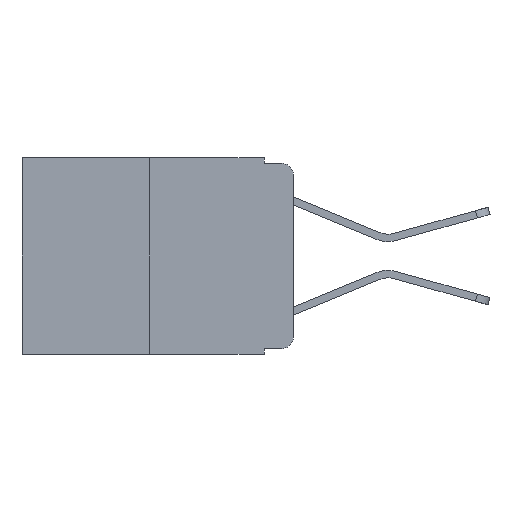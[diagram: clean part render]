
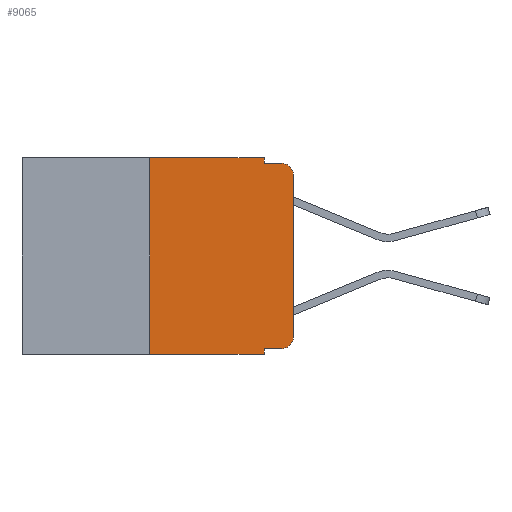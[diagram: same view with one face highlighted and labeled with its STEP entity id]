
A CAD part, left-side view. The second image highlights one B-rep face of the part: STEP entity #9065.
In plain terms, the highlighted planar face has unit normal (-1, 0, 0).
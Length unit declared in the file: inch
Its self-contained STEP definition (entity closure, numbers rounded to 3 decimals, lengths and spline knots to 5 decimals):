
#629 = DIRECTION ( 'NONE',  ( -1., 0., 0. ) ) ;
#925 = LINE ( 'NONE', #5400, #9037 ) ;
#947 = VECTOR ( 'NONE', #1078, 39.37008 ) ;
#1078 = DIRECTION ( 'NONE',  ( 0., 0., -1. ) ) ;
#1231 = VECTOR ( 'NONE', #9733, 39.37008 ) ;
#1536 = CARTESIAN_POINT ( 'NONE',  ( 0., 0.02, -0.03 ) ) ;
#1840 = VECTOR ( 'NONE', #14972, 39.37008 ) ;
#2281 = VERTEX_POINT ( 'NONE', #4823 ) ;
#3013 = CARTESIAN_POINT ( 'NONE',  ( 0., 0.051, 0. ) ) ;
#3278 = DIRECTION ( 'NONE',  ( 0., 0., -1. ) ) ;
#3387 = VERTEX_POINT ( 'NONE', #6013 ) ;
#3464 = LINE ( 'NONE', #14031, #18891 ) ;
#3609 = VERTEX_POINT ( 'NONE', #5540 ) ;
#3781 = CIRCLE ( 'NONE', #15953, 0.02 ) ;
#3854 = VERTEX_POINT ( 'NONE', #15991 ) ;
#3894 = EDGE_CURVE ( 'NONE', #6887, #2281, #3464, .T. ) ;
#3953 = VECTOR ( 'NONE', #13714, 39.37008 ) ;
#4416 = DIRECTION ( 'NONE',  ( 0., -1., 0. ) ) ;
#4648 = VERTEX_POINT ( 'NONE', #9724 ) ;
#4730 = ORIENTED_EDGE ( 'NONE', *, *, #18257, .F. ) ;
#4823 = CARTESIAN_POINT ( 'NONE',  ( 0., 0.051, -0.343 ) ) ;
#4952 = ORIENTED_EDGE ( 'NONE', *, *, #6186, .F. ) ;
#4971 = ORIENTED_EDGE ( 'NONE', *, *, #3894, .T. ) ;
#5252 = DIRECTION ( 'NONE',  ( 0., 0., 1. ) ) ;
#5400 = CARTESIAN_POINT ( 'NONE',  ( 0., 0.051, -0.01 ) ) ;
#5460 = DIRECTION ( 'NONE',  ( 0., -1., 0. ) ) ;
#5540 = CARTESIAN_POINT ( 'NONE',  ( 0., 0.02, -0.333 ) ) ;
#6013 = CARTESIAN_POINT ( 'NONE',  ( 0., 0.051, -0.01 ) ) ;
#6060 = CARTESIAN_POINT ( 'NONE',  ( 0., 0.25, 0. ) ) ;
#6186 = EDGE_CURVE ( 'NONE', #3387, #3854, #925, .T. ) ;
#6706 = ORIENTED_EDGE ( 'NONE', *, *, #17439, .F. ) ;
#6887 = VERTEX_POINT ( 'NONE', #12874 ) ;
#6888 = CARTESIAN_POINT ( 'NONE',  ( 0., 0.051, -0.333 ) ) ;
#7159 = DIRECTION ( 'NONE',  ( 0., 0., -1. ) ) ;
#7448 = VECTOR ( 'NONE', #5252, 39.37008 ) ;
#7503 = CARTESIAN_POINT ( 'NONE',  ( 0., 0.473, 0. ) ) ;
#8225 = CARTESIAN_POINT ( 'NONE',  ( 0., 0.051, -0.333 ) ) ;
#8595 = LINE ( 'NONE', #3013, #3953 ) ;
#8631 = PLANE ( 'NONE',  #9180 ) ;
#9024 = ORIENTED_EDGE ( 'NONE', *, *, #17099, .T. ) ;
#9037 = VECTOR ( 'NONE', #5460, 39.37008 ) ;
#9065 = ADVANCED_FACE ( 'NONE', ( #17195 ), #8631, .F. ) ;
#9180 = AXIS2_PLACEMENT_3D ( 'NONE', #14538, #16006, #7159 ) ;
#9534 = ORIENTED_EDGE ( 'NONE', *, *, #12596, .F. ) ;
#9543 = LINE ( 'NONE', #15046, #947 ) ;
#9634 = CARTESIAN_POINT ( 'NONE',  ( 0., 0., -0.03 ) ) ;
#9724 = CARTESIAN_POINT ( 'NONE',  ( 0., 0., -0.313 ) ) ;
#9733 = DIRECTION ( 'NONE',  ( 0., -1., 0. ) ) ;
#10222 = CARTESIAN_POINT ( 'NONE',  ( 0., 0.051, 0. ) ) ;
#10256 = EDGE_CURVE ( 'NONE', #14194, #3854, #3781, .T. ) ;
#10281 = LINE ( 'NONE', #6060, #1840 ) ;
#10285 = CARTESIAN_POINT ( 'NONE',  ( 0., 0.02, -0.313 ) ) ;
#11759 = DIRECTION ( 'NONE',  ( 0., 0., -1. ) ) ;
#11809 = VECTOR ( 'NONE', #4416, 39.37008 ) ;
#12311 = VERTEX_POINT ( 'NONE', #10222 ) ;
#12346 = EDGE_CURVE ( 'NONE', #3609, #4648, #15278, .T. ) ;
#12493 = DIRECTION ( 'NONE',  ( -1., 0., 0. ) ) ;
#12596 = EDGE_CURVE ( 'NONE', #12311, #3387, #8595, .T. ) ;
#12758 = ORIENTED_EDGE ( 'NONE', *, *, #10256, .T. ) ;
#12771 = CARTESIAN_POINT ( 'NONE',  ( 0., 0., 0. ) ) ;
#12874 = CARTESIAN_POINT ( 'NONE',  ( 0., 0.25, -0.343 ) ) ;
#13230 = ORIENTED_EDGE ( 'NONE', *, *, #18505, .T. ) ;
#13714 = DIRECTION ( 'NONE',  ( 0., 0., -1. ) ) ;
#14031 = CARTESIAN_POINT ( 'NONE',  ( 0., 0.473, -0.343 ) ) ;
#14194 = VERTEX_POINT ( 'NONE', #9634 ) ;
#14538 = CARTESIAN_POINT ( 'NONE',  ( 0., 0.473, 0. ) ) ;
#14972 = DIRECTION ( 'NONE',  ( 0., 0., 1. ) ) ;
#15046 = CARTESIAN_POINT ( 'NONE',  ( 0., 0.051, 0. ) ) ;
#15067 = ORIENTED_EDGE ( 'NONE', *, *, #12346, .T. ) ;
#15278 = CIRCLE ( 'NONE', #17652, 0.02 ) ;
#15627 = VERTEX_POINT ( 'NONE', #6888 ) ;
#15692 = LINE ( 'NONE', #7503, #11809 ) ;
#15775 = LINE ( 'NONE', #12771, #7448 ) ;
#15953 = AXIS2_PLACEMENT_3D ( 'NONE', #1536, #12493, #3278 ) ;
#15991 = CARTESIAN_POINT ( 'NONE',  ( 0., 0.02, -0.01 ) ) ;
#15995 = CARTESIAN_POINT ( 'NONE',  ( 0., 0.25, 0. ) ) ;
#16006 = DIRECTION ( 'NONE',  ( 1., 0., 0. ) ) ;
#16457 = DIRECTION ( 'NONE',  ( 0., -1., 0. ) ) ;
#17099 = EDGE_CURVE ( 'NONE', #4648, #14194, #15775, .T. ) ;
#17195 = FACE_OUTER_BOUND ( 'NONE', #19359, .T. ) ;
#17231 = VERTEX_POINT ( 'NONE', #15995 ) ;
#17439 = EDGE_CURVE ( 'NONE', #6887, #17231, #10281, .T. ) ;
#17525 = ORIENTED_EDGE ( 'NONE', *, *, #19636, .F. ) ;
#17652 = AXIS2_PLACEMENT_3D ( 'NONE', #10285, #629, #11759 ) ;
#17962 = LINE ( 'NONE', #8225, #1231 ) ;
#18257 = EDGE_CURVE ( 'NONE', #15627, #2281, #9543, .T. ) ;
#18505 = EDGE_CURVE ( 'NONE', #15627, #3609, #17962, .T. ) ;
#18891 = VECTOR ( 'NONE', #16457, 39.37008 ) ;
#19359 = EDGE_LOOP ( 'NONE', ( #9024, #12758, #4952, #9534, #17525, #6706, #4971, #4730, #13230, #15067 ) ) ;
#19636 = EDGE_CURVE ( 'NONE', #17231, #12311, #15692, .T. ) ;
